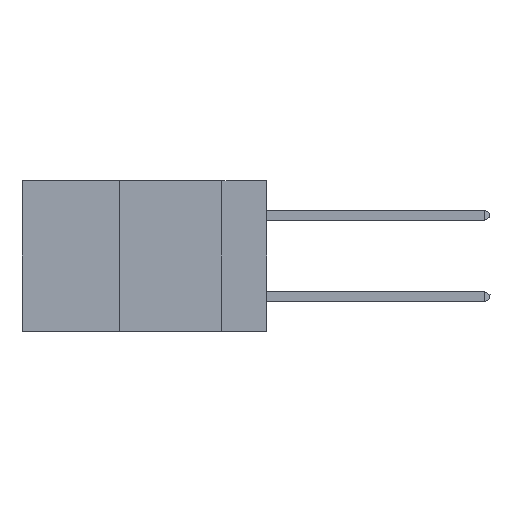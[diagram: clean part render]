
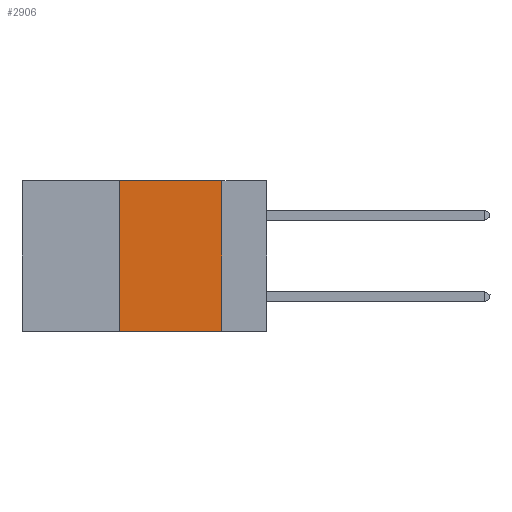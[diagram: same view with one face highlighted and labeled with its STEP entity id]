
A CAD part, left-side view. The second image highlights one B-rep face of the part: STEP entity #2906.
In plain terms, the highlighted planar face has unit normal (-1, 0, 0).
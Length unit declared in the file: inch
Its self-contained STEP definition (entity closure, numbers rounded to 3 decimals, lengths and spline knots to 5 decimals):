
#302 = VECTOR ( 'NONE', #6938, 39.37008 ) ;
#355 = VECTOR ( 'NONE', #1850, 39.37008 ) ;
#963 = CARTESIAN_POINT ( 'NONE',  ( 0., 0.11, 0. ) ) ;
#1184 = ORIENTED_EDGE ( 'NONE', *, *, #7744, .T. ) ;
#1388 = CARTESIAN_POINT ( 'NONE',  ( 0., 0.11, 0. ) ) ;
#1611 = CARTESIAN_POINT ( 'NONE',  ( 0., 0.6, 0. ) ) ;
#1850 = DIRECTION ( 'NONE',  ( 0., -1., 0. ) ) ;
#2489 = LINE ( 'NONE', #1611, #6490 ) ;
#2512 = PLANE ( 'NONE',  #2977 ) ;
#2756 = EDGE_LOOP ( 'NONE', ( #4064, #6848, #6999, #1184 ) ) ;
#2906 = ADVANCED_FACE ( 'NONE', ( #7069 ), #2512, .F. ) ;
#2977 = AXIS2_PLACEMENT_3D ( 'NONE', #6350, #4152, #9224 ) ;
#3185 = EDGE_CURVE ( 'NONE', #3705, #5333, #2489, .T. ) ;
#3705 = VERTEX_POINT ( 'NONE', #3775 ) ;
#3775 = CARTESIAN_POINT ( 'NONE',  ( 0., 0.36, 0. ) ) ;
#4008 = DIRECTION ( 'NONE',  ( 0., 0., -1. ) ) ;
#4064 = ORIENTED_EDGE ( 'NONE', *, *, #5136, .F. ) ;
#4067 = CARTESIAN_POINT ( 'NONE',  ( 0., 0.36, 0. ) ) ;
#4152 = DIRECTION ( 'NONE',  ( 1., 0., 0. ) ) ;
#4650 = EDGE_CURVE ( 'NONE', #7979, #3705, #4780, .T. ) ;
#4671 = LINE ( 'NONE', #963, #6410 ) ;
#4780 = LINE ( 'NONE', #4067, #302 ) ;
#4896 = CARTESIAN_POINT ( 'NONE',  ( 0., 0.11, -0.37 ) ) ;
#5136 = EDGE_CURVE ( 'NONE', #5333, #8795, #4671, .T. ) ;
#5333 = VERTEX_POINT ( 'NONE', #1388 ) ;
#6350 = CARTESIAN_POINT ( 'NONE',  ( 0., 0.6, 0. ) ) ;
#6410 = VECTOR ( 'NONE', #4008, 39.37008 ) ;
#6490 = VECTOR ( 'NONE', #8298, 39.37008 ) ;
#6848 = ORIENTED_EDGE ( 'NONE', *, *, #3185, .F. ) ;
#6938 = DIRECTION ( 'NONE',  ( 0., 0., 1. ) ) ;
#6999 = ORIENTED_EDGE ( 'NONE', *, *, #4650, .F. ) ;
#7069 = FACE_OUTER_BOUND ( 'NONE', #2756, .T. ) ;
#7658 = LINE ( 'NONE', #8439, #355 ) ;
#7744 = EDGE_CURVE ( 'NONE', #7979, #8795, #7658, .T. ) ;
#7979 = VERTEX_POINT ( 'NONE', #8457 ) ;
#8298 = DIRECTION ( 'NONE',  ( 0., -1., 0. ) ) ;
#8439 = CARTESIAN_POINT ( 'NONE',  ( 0., 0.6, -0.37 ) ) ;
#8457 = CARTESIAN_POINT ( 'NONE',  ( 0., 0.36, -0.37 ) ) ;
#8795 = VERTEX_POINT ( 'NONE', #4896 ) ;
#9224 = DIRECTION ( 'NONE',  ( 0., 0., -1. ) ) ;
